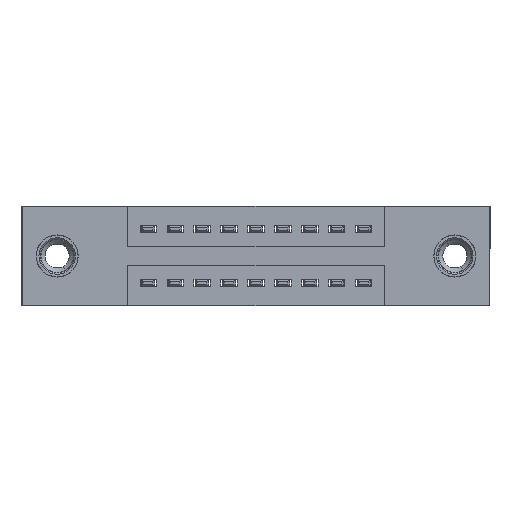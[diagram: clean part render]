
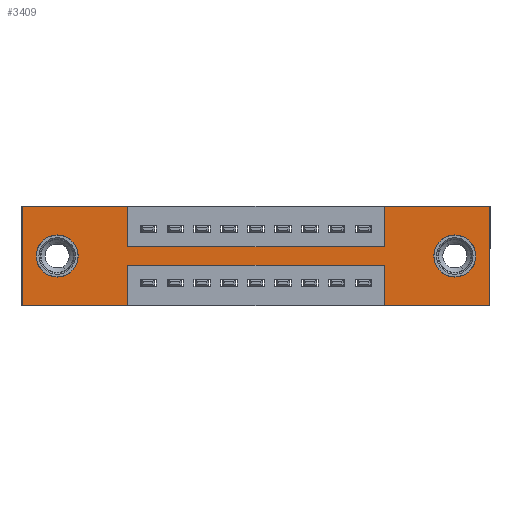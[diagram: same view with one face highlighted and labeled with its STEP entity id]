
A CAD part, front view. The second image highlights one B-rep face of the part: STEP entity #3409.
In plain terms, the highlighted planar face has unit normal (0, -1, 0).
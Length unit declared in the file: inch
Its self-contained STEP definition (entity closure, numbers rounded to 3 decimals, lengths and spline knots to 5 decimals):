
#28 = CARTESIAN_POINT ( 'NONE',  ( 1.3425, 0., -0.37 ) ) ;
#38 = DIRECTION ( 'NONE',  ( 1., 0., 0. ) ) ;
#274 = VECTOR ( 'NONE', #4644, 39.37008 ) ;
#383 = CARTESIAN_POINT ( 'NONE',  ( 0.3925, 0., -0.15 ) ) ;
#409 = ORIENTED_EDGE ( 'NONE', *, *, #572, .F. ) ;
#435 = EDGE_CURVE ( 'NONE', #8322, #11137, #1931, .T. ) ;
#459 = LINE ( 'NONE', #10891, #274 ) ;
#469 = VERTEX_POINT ( 'NONE', #481 ) ;
#481 = CARTESIAN_POINT ( 'NONE',  ( 0., 0., 0. ) ) ;
#536 = CARTESIAN_POINT ( 'NONE',  ( 1.3425, 0., -0.37 ) ) ;
#572 = EDGE_CURVE ( 'NONE', #11137, #11856, #645, .T. ) ;
#645 = LINE ( 'NONE', #2739, #6902 ) ;
#765 = VECTOR ( 'NONE', #3023, 39.37008 ) ;
#794 = LINE ( 'NONE', #8626, #1111 ) ;
#922 = VERTEX_POINT ( 'NONE', #4098 ) ;
#923 = DIRECTION ( 'NONE',  ( 0., 0., -1. ) ) ;
#965 = CARTESIAN_POINT ( 'NONE',  ( 1.605, 0., -0.185 ) ) ;
#1028 = CARTESIAN_POINT ( 'NONE',  ( 0.13, 0., -0.185 ) ) ;
#1111 = VECTOR ( 'NONE', #10694, 39.37008 ) ;
#1226 = VECTOR ( 'NONE', #9718, 39.37008 ) ;
#1335 = EDGE_CURVE ( 'NONE', #11629, #11981, #13339, .T. ) ;
#1350 = CARTESIAN_POINT ( 'NONE',  ( 0., 0., -0.37 ) ) ;
#1518 = EDGE_LOOP ( 'NONE', ( #2373, #1971 ) ) ;
#1618 = VECTOR ( 'NONE', #9281, 39.37008 ) ;
#1670 = ORIENTED_EDGE ( 'NONE', *, *, #2249, .F. ) ;
#1931 = LINE ( 'NONE', #11467, #1618 ) ;
#1971 = ORIENTED_EDGE ( 'NONE', *, *, #3358, .T. ) ;
#2025 = ORIENTED_EDGE ( 'NONE', *, *, #2422, .F. ) ;
#2034 = VERTEX_POINT ( 'NONE', #6277 ) ;
#2066 = AXIS2_PLACEMENT_3D ( 'NONE', #3344, #11749, #3483 ) ;
#2249 = EDGE_CURVE ( 'NONE', #469, #8322, #459, .T. ) ;
#2368 = VECTOR ( 'NONE', #6241, 39.37008 ) ;
#2373 = ORIENTED_EDGE ( 'NONE', *, *, #8398, .T. ) ;
#2380 = ORIENTED_EDGE ( 'NONE', *, *, #3189, .F. ) ;
#2422 = EDGE_CURVE ( 'NONE', #4596, #10961, #11507, .T. ) ;
#2438 = ORIENTED_EDGE ( 'NONE', *, *, #5681, .F. ) ;
#2660 = AXIS2_PLACEMENT_3D ( 'NONE', #10372, #4201, #10506 ) ;
#2684 = LINE ( 'NONE', #9283, #1226 ) ;
#2739 = CARTESIAN_POINT ( 'NONE',  ( 0.3925, 0., -0.15 ) ) ;
#2781 = CARTESIAN_POINT ( 'NONE',  ( 0.13, 0., -0.107 ) ) ;
#2786 = DIRECTION ( 'NONE',  ( 1., 0., 0. ) ) ;
#3015 = ORIENTED_EDGE ( 'NONE', *, *, #8997, .F. ) ;
#3023 = DIRECTION ( 'NONE',  ( 0., 0., -1. ) ) ;
#3047 = CARTESIAN_POINT ( 'NONE',  ( 1.3425, 0., -0.22 ) ) ;
#3189 = EDGE_CURVE ( 'NONE', #922, #6403, #6234, .T. ) ;
#3191 = EDGE_CURVE ( 'NONE', #4226, #922, #3657, .T. ) ;
#3295 = DIRECTION ( 'NONE',  ( 0., 0., -1. ) ) ;
#3344 = CARTESIAN_POINT ( 'NONE',  ( 0., 0., -0.37 ) ) ;
#3358 = EDGE_CURVE ( 'NONE', #7608, #7524, #9147, .T. ) ;
#3409 = ADVANCED_FACE ( 'NONE', ( #4456, #10631, #7856 ), #5552, .T. ) ;
#3483 = DIRECTION ( 'NONE',  ( 0., 0., -1. ) ) ;
#3657 = LINE ( 'NONE', #9161, #4140 ) ;
#3742 = DIRECTION ( 'NONE',  ( 0., 1., 0. ) ) ;
#3848 = DIRECTION ( 'NONE',  ( 0., 0., -1. ) ) ;
#3934 = CARTESIAN_POINT ( 'NONE',  ( 0.3925, 0., -0.37 ) ) ;
#4098 = CARTESIAN_POINT ( 'NONE',  ( 1.735, 0., 0. ) ) ;
#4140 = VECTOR ( 'NONE', #38, 39.37008 ) ;
#4201 = DIRECTION ( 'NONE',  ( 0., 1., 0. ) ) ;
#4226 = VERTEX_POINT ( 'NONE', #11595 ) ;
#4231 = EDGE_CURVE ( 'NONE', #11981, #11629, #5394, .T. ) ;
#4395 = ORIENTED_EDGE ( 'NONE', *, *, #9958, .F. ) ;
#4456 = FACE_BOUND ( 'NONE', #11590, .T. ) ;
#4596 = VERTEX_POINT ( 'NONE', #536 ) ;
#4644 = DIRECTION ( 'NONE',  ( 1., 0., 0. ) ) ;
#5048 = VECTOR ( 'NONE', #7526, 39.37008 ) ;
#5093 = DIRECTION ( 'NONE',  ( 0., 0., 1. ) ) ;
#5127 = CARTESIAN_POINT ( 'NONE',  ( 1.605, 0., -0.263 ) ) ;
#5357 = LINE ( 'NONE', #1350, #5048 ) ;
#5394 = CIRCLE ( 'NONE', #10855, 0.078 ) ;
#5552 = PLANE ( 'NONE',  #2066 ) ;
#5638 = CARTESIAN_POINT ( 'NONE',  ( 1.605, 0., -0.107 ) ) ;
#5681 = EDGE_CURVE ( 'NONE', #6403, #4596, #5357, .T. ) ;
#5974 = EDGE_LOOP ( 'NONE', ( #4395, #8923, #2025, #2438, #2380, #7656, #6097, #409, #8551, #1670, #3015, #8509 ) ) ;
#6033 = VERTEX_POINT ( 'NONE', #7535 ) ;
#6097 = ORIENTED_EDGE ( 'NONE', *, *, #6700, .F. ) ;
#6234 = LINE ( 'NONE', #9296, #765 ) ;
#6241 = DIRECTION ( 'NONE',  ( 0., 0., 1. ) ) ;
#6277 = CARTESIAN_POINT ( 'NONE',  ( 0.3925, 0., -0.37 ) ) ;
#6403 = VERTEX_POINT ( 'NONE', #7584 ) ;
#6700 = EDGE_CURVE ( 'NONE', #11856, #4226, #12699, .T. ) ;
#6773 = LINE ( 'NONE', #3934, #11218 ) ;
#6902 = VECTOR ( 'NONE', #2786, 39.37008 ) ;
#7062 = ORIENTED_EDGE ( 'NONE', *, *, #4231, .T. ) ;
#7124 = CIRCLE ( 'NONE', #2660, 0.078 ) ;
#7283 = VECTOR ( 'NONE', #9184, 39.37008 ) ;
#7524 = VERTEX_POINT ( 'NONE', #2781 ) ;
#7526 = DIRECTION ( 'NONE',  ( -1., 0., 0. ) ) ;
#7535 = CARTESIAN_POINT ( 'NONE',  ( 0., 0., -0.37 ) ) ;
#7584 = CARTESIAN_POINT ( 'NONE',  ( 1.735, 0., -0.37 ) ) ;
#7608 = VERTEX_POINT ( 'NONE', #11333 ) ;
#7656 = ORIENTED_EDGE ( 'NONE', *, *, #3191, .F. ) ;
#7856 = FACE_OUTER_BOUND ( 'NONE', #5974, .T. ) ;
#8104 = CARTESIAN_POINT ( 'NONE',  ( 0., 0., 0. ) ) ;
#8321 = DIRECTION ( 'NONE',  ( 0., 0., 1. ) ) ;
#8322 = VERTEX_POINT ( 'NONE', #12482 ) ;
#8398 = EDGE_CURVE ( 'NONE', #7524, #7608, #7124, .T. ) ;
#8509 = ORIENTED_EDGE ( 'NONE', *, *, #10502, .F. ) ;
#8551 = ORIENTED_EDGE ( 'NONE', *, *, #435, .F. ) ;
#8626 = CARTESIAN_POINT ( 'NONE',  ( 0., 0., -0.37 ) ) ;
#8923 = ORIENTED_EDGE ( 'NONE', *, *, #12424, .F. ) ;
#8961 = AXIS2_PLACEMENT_3D ( 'NONE', #965, #10233, #923 ) ;
#8997 = EDGE_CURVE ( 'NONE', #6033, #469, #12230, .T. ) ;
#9147 = CIRCLE ( 'NONE', #13305, 0.078 ) ;
#9161 = CARTESIAN_POINT ( 'NONE',  ( 0., 0., 0. ) ) ;
#9184 = DIRECTION ( 'NONE',  ( 0., 0., 1. ) ) ;
#9281 = DIRECTION ( 'NONE',  ( 0., 0., -1. ) ) ;
#9283 = CARTESIAN_POINT ( 'NONE',  ( 0.3925, 0., -0.22 ) ) ;
#9296 = CARTESIAN_POINT ( 'NONE',  ( 1.735, 0., 0. ) ) ;
#9476 = DIRECTION ( 'NONE',  ( 0., 1., 0. ) ) ;
#9650 = ORIENTED_EDGE ( 'NONE', *, *, #1335, .T. ) ;
#9698 = VECTOR ( 'NONE', #5093, 39.37008 ) ;
#9718 = DIRECTION ( 'NONE',  ( -1., 0., 0. ) ) ;
#9958 = EDGE_CURVE ( 'NONE', #10276, #2034, #6773, .T. ) ;
#10233 = DIRECTION ( 'NONE',  ( 0., 1., 0. ) ) ;
#10276 = VERTEX_POINT ( 'NONE', #12350 ) ;
#10372 = CARTESIAN_POINT ( 'NONE',  ( 0.13, 0., -0.185 ) ) ;
#10502 = EDGE_CURVE ( 'NONE', #2034, #6033, #794, .T. ) ;
#10506 = DIRECTION ( 'NONE',  ( 0., 0., 1. ) ) ;
#10631 = FACE_BOUND ( 'NONE', #1518, .T. ) ;
#10694 = DIRECTION ( 'NONE',  ( -1., 0., 0. ) ) ;
#10855 = AXIS2_PLACEMENT_3D ( 'NONE', #11730, #9476, #3295 ) ;
#10891 = CARTESIAN_POINT ( 'NONE',  ( 0., 0., 0. ) ) ;
#10961 = VERTEX_POINT ( 'NONE', #3047 ) ;
#11137 = VERTEX_POINT ( 'NONE', #383 ) ;
#11218 = VECTOR ( 'NONE', #3848, 39.37008 ) ;
#11333 = CARTESIAN_POINT ( 'NONE',  ( 0.13, 0., -0.263 ) ) ;
#11365 = CARTESIAN_POINT ( 'NONE',  ( 1.3425, 0., 0. ) ) ;
#11467 = CARTESIAN_POINT ( 'NONE',  ( 0.3925, 0., 0. ) ) ;
#11507 = LINE ( 'NONE', #28, #2368 ) ;
#11590 = EDGE_LOOP ( 'NONE', ( #9650, #7062 ) ) ;
#11595 = CARTESIAN_POINT ( 'NONE',  ( 1.3425, 0., 0. ) ) ;
#11629 = VERTEX_POINT ( 'NONE', #5638 ) ;
#11730 = CARTESIAN_POINT ( 'NONE',  ( 1.605, 0., -0.185 ) ) ;
#11749 = DIRECTION ( 'NONE',  ( 0., -1., 0. ) ) ;
#11856 = VERTEX_POINT ( 'NONE', #13151 ) ;
#11981 = VERTEX_POINT ( 'NONE', #5127 ) ;
#12230 = LINE ( 'NONE', #8104, #7283 ) ;
#12350 = CARTESIAN_POINT ( 'NONE',  ( 0.3925, 0., -0.22 ) ) ;
#12424 = EDGE_CURVE ( 'NONE', #10961, #10276, #2684, .T. ) ;
#12482 = CARTESIAN_POINT ( 'NONE',  ( 0.3925, 0., 0. ) ) ;
#12699 = LINE ( 'NONE', #11365, #9698 ) ;
#13151 = CARTESIAN_POINT ( 'NONE',  ( 1.3425, 0., -0.15 ) ) ;
#13305 = AXIS2_PLACEMENT_3D ( 'NONE', #1028, #3742, #8321 ) ;
#13339 = CIRCLE ( 'NONE', #8961, 0.078 ) ;
